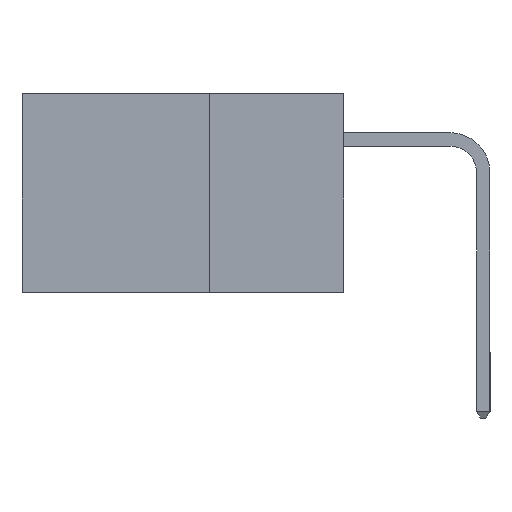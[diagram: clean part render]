
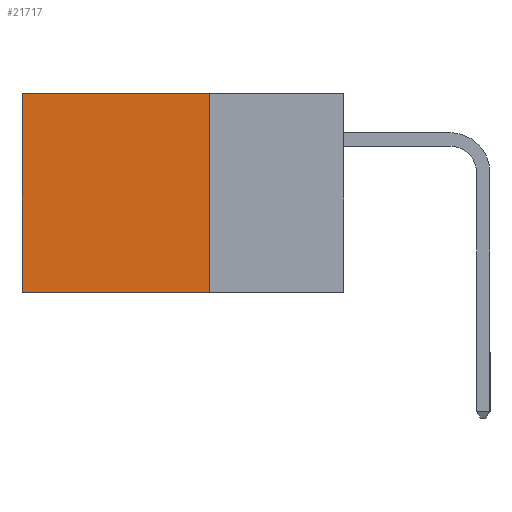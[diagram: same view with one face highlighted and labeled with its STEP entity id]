
A CAD part, left-side view. The second image highlights one B-rep face of the part: STEP entity #21717.
In plain terms, the highlighted planar face has unit normal (-1, 0, 0).
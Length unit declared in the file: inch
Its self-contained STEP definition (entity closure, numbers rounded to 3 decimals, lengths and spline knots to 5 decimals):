
#439 = EDGE_CURVE ( 'NONE', #17483, #18227, #7066, .T. ) ;
#1559 = VECTOR ( 'NONE', #17925, 39.37008 ) ;
#2115 = CARTESIAN_POINT ( 'NONE',  ( 0.298, 0.6, 0. ) ) ;
#3197 = CARTESIAN_POINT ( 'NONE',  ( 0.298, 0.25, 0. ) ) ;
#3444 = VERTEX_POINT ( 'NONE', #18577 ) ;
#3785 = ORIENTED_EDGE ( 'NONE', *, *, #5271, .F. ) ;
#4115 = DIRECTION ( 'NONE',  ( 0., 0., -1. ) ) ;
#4184 = VECTOR ( 'NONE', #9688, 39.37008 ) ;
#4209 = CARTESIAN_POINT ( 'NONE',  ( 0.298, 0.25, -0.37 ) ) ;
#4768 = LINE ( 'NONE', #4209, #4184 ) ;
#5271 = EDGE_CURVE ( 'NONE', #3444, #22014, #21568, .T. ) ;
#6074 = EDGE_CURVE ( 'NONE', #3444, #17483, #15658, .T. ) ;
#6134 = DIRECTION ( 'NONE',  ( 0., 0., -1. ) ) ;
#6369 = CARTESIAN_POINT ( 'NONE',  ( 0.298, 0.6, 0. ) ) ;
#6958 = CARTESIAN_POINT ( 'NONE',  ( 0.298, 0.6, -0.37 ) ) ;
#7066 = LINE ( 'NONE', #6369, #9036 ) ;
#9036 = VECTOR ( 'NONE', #6134, 39.37008 ) ;
#9183 = EDGE_LOOP ( 'NONE', ( #11575, #10534, #3785, #15368 ) ) ;
#9391 = CARTESIAN_POINT ( 'NONE',  ( 0.298, 0.25, 0. ) ) ;
#9688 = DIRECTION ( 'NONE',  ( 0., 1., 0. ) ) ;
#10534 = ORIENTED_EDGE ( 'NONE', *, *, #14420, .F. ) ;
#11221 = DIRECTION ( 'NONE',  ( 0., 1., 0. ) ) ;
#11575 = ORIENTED_EDGE ( 'NONE', *, *, #439, .T. ) ;
#13483 = CARTESIAN_POINT ( 'NONE',  ( 0.298, 0.25, 0. ) ) ;
#14420 = EDGE_CURVE ( 'NONE', #22014, #18227, #4768, .T. ) ;
#15283 = DIRECTION ( 'NONE',  ( 1., 0., 0. ) ) ;
#15368 = ORIENTED_EDGE ( 'NONE', *, *, #6074, .T. ) ;
#15658 = LINE ( 'NONE', #9391, #19831 ) ;
#16146 = FACE_OUTER_BOUND ( 'NONE', #9183, .T. ) ;
#16391 = PLANE ( 'NONE',  #22042 ) ;
#17483 = VERTEX_POINT ( 'NONE', #2115 ) ;
#17925 = DIRECTION ( 'NONE',  ( 0., 0., -1. ) ) ;
#18227 = VERTEX_POINT ( 'NONE', #6958 ) ;
#18577 = CARTESIAN_POINT ( 'NONE',  ( 0.298, 0.25, 0. ) ) ;
#19302 = CARTESIAN_POINT ( 'NONE',  ( 0.298, 0.25, -0.37 ) ) ;
#19831 = VECTOR ( 'NONE', #11221, 39.37008 ) ;
#21568 = LINE ( 'NONE', #3197, #1559 ) ;
#21717 = ADVANCED_FACE ( 'NONE', ( #16146 ), #16391, .F. ) ;
#22014 = VERTEX_POINT ( 'NONE', #19302 ) ;
#22042 = AXIS2_PLACEMENT_3D ( 'NONE', #13483, #15283, #4115 ) ;
